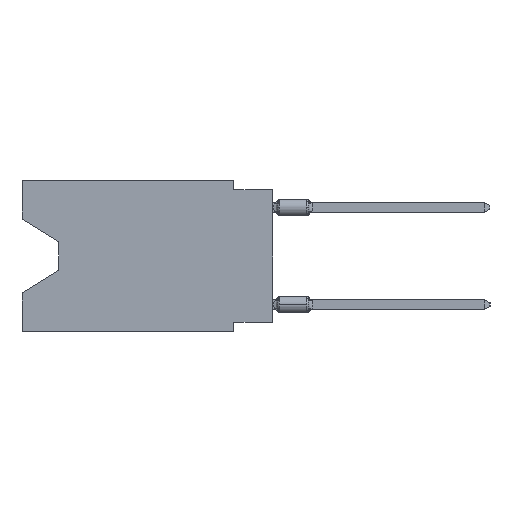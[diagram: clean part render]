
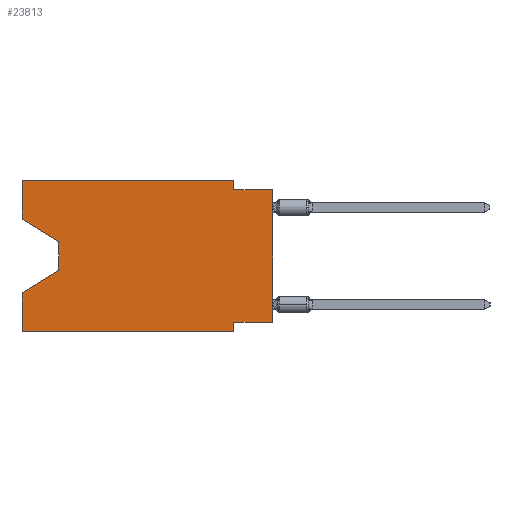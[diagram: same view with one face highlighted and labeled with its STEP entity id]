
A CAD part, left-side view. The second image highlights one B-rep face of the part: STEP entity #23813.
In plain terms, the highlighted planar face has unit normal (-1, 0, 0).
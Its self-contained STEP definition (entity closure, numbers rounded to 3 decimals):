
#530 = DIRECTION ( 'NONE',  ( 1., 0., 0. ) ) ;
#658 = ORIENTED_EDGE ( 'NONE', *, *, #18542, .T. ) ;
#728 = VERTEX_POINT ( 'NONE', #14886 ) ;
#1070 = EDGE_CURVE ( 'NONE', #9315, #12119, #46962, .T. ) ;
#2246 = ORIENTED_EDGE ( 'NONE', *, *, #46357, .T. ) ;
#2437 = VECTOR ( 'NONE', #2799, 1000. ) ;
#2614 = VECTOR ( 'NONE', #13612, 1000. ) ;
#2799 = DIRECTION ( 'NONE',  ( 0., -1., 0. ) ) ;
#3305 = DIRECTION ( 'NONE',  ( 0., 1., 0. ) ) ;
#4150 = LINE ( 'NONE', #38469, #23917 ) ;
#4442 = DIRECTION ( 'NONE',  ( 0., 0., 1. ) ) ;
#5569 = DIRECTION ( 'NONE',  ( 0., -1., 0. ) ) ;
#7351 = ORIENTED_EDGE ( 'NONE', *, *, #51622, .F. ) ;
#9258 = ORIENTED_EDGE ( 'NONE', *, *, #19561, .F. ) ;
#9315 = VERTEX_POINT ( 'NONE', #25091 ) ;
#9756 = LINE ( 'NONE', #19998, #21861 ) ;
#11165 = CARTESIAN_POINT ( 'NONE',  ( 0., 16.383, -9.906 ) ) ;
#11856 = ORIENTED_EDGE ( 'NONE', *, *, #1070, .F. ) ;
#11998 = VERTEX_POINT ( 'NONE', #49030 ) ;
#12119 = VERTEX_POINT ( 'NONE', #16568 ) ;
#13433 = LINE ( 'NONE', #33010, #21109 ) ;
#13612 = DIRECTION ( 'NONE',  ( 0., -1., 0. ) ) ;
#14318 = FACE_OUTER_BOUND ( 'NONE', #33602, .T. ) ;
#14635 = DIRECTION ( 'NONE',  ( 0., 0., -1. ) ) ;
#14886 = CARTESIAN_POINT ( 'NONE',  ( 0., 2.54, -0.635 ) ) ;
#15406 = LINE ( 'NONE', #40141, #47469 ) ;
#15640 = CARTESIAN_POINT ( 'NONE',  ( 0., 16.383, -7.36 ) ) ;
#16493 = CARTESIAN_POINT ( 'NONE',  ( 0., 2.54, 0. ) ) ;
#16568 = CARTESIAN_POINT ( 'NONE',  ( 0., 2.54, -9.271 ) ) ;
#18375 = CARTESIAN_POINT ( 'NONE',  ( 0., 0., -9.271 ) ) ;
#18542 = EDGE_CURVE ( 'NONE', #11998, #22460, #29808, .T. ) ;
#18700 = EDGE_CURVE ( 'NONE', #49219, #61510, #57587, .T. ) ;
#18842 = CARTESIAN_POINT ( 'NONE',  ( 0., 2.54, 0. ) ) ;
#19561 = EDGE_CURVE ( 'NONE', #23483, #22460, #42374, .T. ) ;
#19801 = ORIENTED_EDGE ( 'NONE', *, *, #45751, .T. ) ;
#19998 = CARTESIAN_POINT ( 'NONE',  ( 0., 0., -0.635 ) ) ;
#20167 = CARTESIAN_POINT ( 'NONE',  ( 0., 2.54, -9.906 ) ) ;
#20982 = LINE ( 'NONE', #16493, #34628 ) ;
#21109 = VECTOR ( 'NONE', #4442, 1000. ) ;
#21704 = CARTESIAN_POINT ( 'NONE',  ( 0., 16.383, -2.546 ) ) ;
#21861 = VECTOR ( 'NONE', #5569, 1000. ) ;
#22460 = VERTEX_POINT ( 'NONE', #15640 ) ;
#22653 = LINE ( 'NONE', #51531, #59835 ) ;
#23483 = VERTEX_POINT ( 'NONE', #39754 ) ;
#23714 = VERTEX_POINT ( 'NONE', #33284 ) ;
#23813 = ADVANCED_FACE ( 'NONE', ( #14318 ), #24289, .F. ) ;
#23917 = VECTOR ( 'NONE', #58056, 1000. ) ;
#24289 = PLANE ( 'NONE',  #30756 ) ;
#24610 = ORIENTED_EDGE ( 'NONE', *, *, #44882, .F. ) ;
#24668 = DIRECTION ( 'NONE',  ( 0., 0.855, -0.519 ) ) ;
#25091 = CARTESIAN_POINT ( 'NONE',  ( 0., 0., -9.271 ) ) ;
#26261 = DIRECTION ( 'NONE',  ( 0., -0.855, -0.519 ) ) ;
#26562 = ORIENTED_EDGE ( 'NONE', *, *, #18700, .F. ) ;
#28444 = EDGE_CURVE ( 'NONE', #37777, #41118, #55136, .T. ) ;
#29808 = LINE ( 'NONE', #59319, #51723 ) ;
#30756 = AXIS2_PLACEMENT_3D ( 'NONE', #49620, #530, #14635 ) ;
#33010 = CARTESIAN_POINT ( 'NONE',  ( 0., 16.383, 0. ) ) ;
#33284 = CARTESIAN_POINT ( 'NONE',  ( 0., 0., -0.635 ) ) ;
#33602 = EDGE_LOOP ( 'NONE', ( #49549, #62222, #658, #9258, #2246, #24610, #11856, #19801, #7351, #40848, #26562, #47003 ) ) ;
#34628 = VECTOR ( 'NONE', #55350, 1000. ) ;
#35095 = EDGE_CURVE ( 'NONE', #37777, #49219, #13433, .T. ) ;
#35865 = LINE ( 'NONE', #11165, #2437 ) ;
#37373 = CARTESIAN_POINT ( 'NONE',  ( 0., 16.383, -2.546 ) ) ;
#37532 = DIRECTION ( 'NONE',  ( 0., 0., 1. ) ) ;
#37777 = VERTEX_POINT ( 'NONE', #21704 ) ;
#37901 = CARTESIAN_POINT ( 'NONE',  ( 0., 13.97, -4.013 ) ) ;
#38469 = CARTESIAN_POINT ( 'NONE',  ( 0., 13.97, -4.013 ) ) ;
#39321 = EDGE_CURVE ( 'NONE', #61510, #728, #20982, .T. ) ;
#39754 = CARTESIAN_POINT ( 'NONE',  ( 0., 16.383, -9.906 ) ) ;
#40141 = CARTESIAN_POINT ( 'NONE',  ( 0., 0., 0. ) ) ;
#40848 = ORIENTED_EDGE ( 'NONE', *, *, #39321, .F. ) ;
#41118 = VERTEX_POINT ( 'NONE', #37901 ) ;
#42374 = LINE ( 'NONE', #61930, #56951 ) ;
#44882 = EDGE_CURVE ( 'NONE', #12119, #54001, #22653, .T. ) ;
#45676 = VECTOR ( 'NONE', #26261, 1000. ) ;
#45751 = EDGE_CURVE ( 'NONE', #9315, #23714, #15406, .T. ) ;
#46041 = EDGE_CURVE ( 'NONE', #41118, #11998, #4150, .T. ) ;
#46357 = EDGE_CURVE ( 'NONE', #23483, #54001, #35865, .T. ) ;
#46962 = LINE ( 'NONE', #18375, #55137 ) ;
#47003 = ORIENTED_EDGE ( 'NONE', *, *, #35095, .F. ) ;
#47469 = VECTOR ( 'NONE', #49449, 1000. ) ;
#47638 = CARTESIAN_POINT ( 'NONE',  ( 0., 16.383, 0. ) ) ;
#49030 = CARTESIAN_POINT ( 'NONE',  ( 0., 13.97, -5.893 ) ) ;
#49219 = VERTEX_POINT ( 'NONE', #57651 ) ;
#49449 = DIRECTION ( 'NONE',  ( 0., 0., 1. ) ) ;
#49549 = ORIENTED_EDGE ( 'NONE', *, *, #28444, .T. ) ;
#49620 = CARTESIAN_POINT ( 'NONE',  ( 0., 16.383, 0. ) ) ;
#51226 = DIRECTION ( 'NONE',  ( 0., 0., -1. ) ) ;
#51531 = CARTESIAN_POINT ( 'NONE',  ( 0., 2.54, -9.906 ) ) ;
#51622 = EDGE_CURVE ( 'NONE', #728, #23714, #9756, .T. ) ;
#51723 = VECTOR ( 'NONE', #24668, 1000. ) ;
#54001 = VERTEX_POINT ( 'NONE', #20167 ) ;
#55136 = LINE ( 'NONE', #37373, #45676 ) ;
#55137 = VECTOR ( 'NONE', #3305, 1000. ) ;
#55350 = DIRECTION ( 'NONE',  ( 0., 0., -1. ) ) ;
#56951 = VECTOR ( 'NONE', #37532, 1000. ) ;
#57587 = LINE ( 'NONE', #47638, #2614 ) ;
#57651 = CARTESIAN_POINT ( 'NONE',  ( 0., 16.383, 0. ) ) ;
#58056 = DIRECTION ( 'NONE',  ( 0., 0., -1. ) ) ;
#59319 = CARTESIAN_POINT ( 'NONE',  ( 0., 13.97, -5.893 ) ) ;
#59835 = VECTOR ( 'NONE', #51226, 1000. ) ;
#61510 = VERTEX_POINT ( 'NONE', #18842 ) ;
#61930 = CARTESIAN_POINT ( 'NONE',  ( 0., 16.383, 0. ) ) ;
#62222 = ORIENTED_EDGE ( 'NONE', *, *, #46041, .T. ) ;
